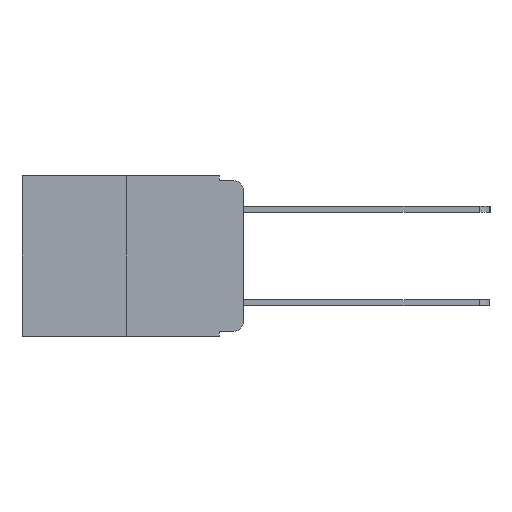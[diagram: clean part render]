
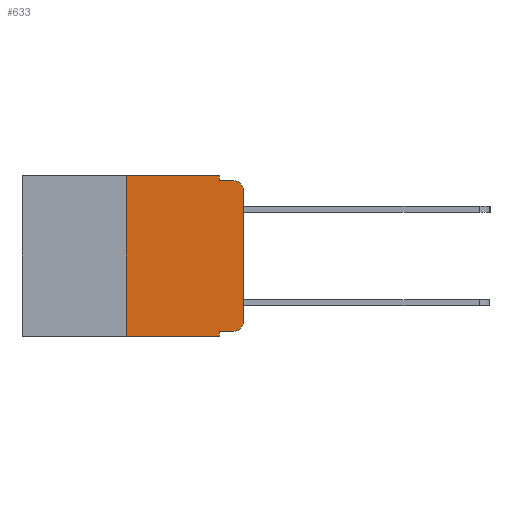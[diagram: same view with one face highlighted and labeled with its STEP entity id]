
A CAD part, left-side view. The second image highlights one B-rep face of the part: STEP entity #633.
In plain terms, the highlighted planar face has unit normal (-1, 0, 0).
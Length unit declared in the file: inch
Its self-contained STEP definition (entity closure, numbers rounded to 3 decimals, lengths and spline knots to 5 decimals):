
#31 = DIRECTION ( 'NONE',  ( 0., 0., -1. ) ) ;
#54 = DIRECTION ( 'NONE',  ( -1., 0., 0. ) ) ;
#389 = CARTESIAN_POINT ( 'NONE',  ( 0., 0.051, -0.333 ) ) ;
#633 = ADVANCED_FACE ( 'NONE', ( #2330 ), #4929, .F. ) ;
#895 = ORIENTED_EDGE ( 'NONE', *, *, #9284, .T. ) ;
#1005 = VERTEX_POINT ( 'NONE', #10512 ) ;
#1057 = ORIENTED_EDGE ( 'NONE', *, *, #10213, .T. ) ;
#1192 = CARTESIAN_POINT ( 'NONE',  ( 0., 0.051, 0. ) ) ;
#1267 = CARTESIAN_POINT ( 'NONE',  ( 0., 0.473, 0. ) ) ;
#1302 = VECTOR ( 'NONE', #1320, 39.37008 ) ;
#1320 = DIRECTION ( 'NONE',  ( 0., -1., 0. ) ) ;
#1490 = ORIENTED_EDGE ( 'NONE', *, *, #11199, .F. ) ;
#1569 = EDGE_CURVE ( 'NONE', #8359, #9452, #6798, .T. ) ;
#1632 = CARTESIAN_POINT ( 'NONE',  ( 0., 0.051, -0.343 ) ) ;
#1919 = ORIENTED_EDGE ( 'NONE', *, *, #7229, .T. ) ;
#2298 = VERTEX_POINT ( 'NONE', #8147 ) ;
#2330 = FACE_OUTER_BOUND ( 'NONE', #6310, .T. ) ;
#2711 = VERTEX_POINT ( 'NONE', #11053 ) ;
#2845 = CARTESIAN_POINT ( 'NONE',  ( 0., 0.02, -0.03 ) ) ;
#3116 = VECTOR ( 'NONE', #3587, 39.37008 ) ;
#3314 = DIRECTION ( 'NONE',  ( 0., 0., -1. ) ) ;
#3316 = DIRECTION ( 'NONE',  ( 1., 0., 0. ) ) ;
#3587 = DIRECTION ( 'NONE',  ( 0., -1., 0. ) ) ;
#3621 = LINE ( 'NONE', #7138, #10541 ) ;
#3807 = DIRECTION ( 'NONE',  ( 0., 0., -1. ) ) ;
#3878 = CIRCLE ( 'NONE', #7748, 0.02 ) ;
#3996 = LINE ( 'NONE', #1267, #10617 ) ;
#4294 = ORIENTED_EDGE ( 'NONE', *, *, #10607, .F. ) ;
#4360 = CARTESIAN_POINT ( 'NONE',  ( 0., 0., -0.313 ) ) ;
#4383 = ORIENTED_EDGE ( 'NONE', *, *, #5489, .T. ) ;
#4604 = EDGE_CURVE ( 'NONE', #1005, #2711, #3621, .T. ) ;
#4820 = DIRECTION ( 'NONE',  ( 0., 0., 1. ) ) ;
#4922 = VERTEX_POINT ( 'NONE', #10764 ) ;
#4929 = PLANE ( 'NONE',  #8745 ) ;
#5046 = VECTOR ( 'NONE', #6000, 39.37008 ) ;
#5053 = LINE ( 'NONE', #1192, #9042 ) ;
#5391 = LINE ( 'NONE', #9741, #10130 ) ;
#5489 = EDGE_CURVE ( 'NONE', #9452, #8325, #3878, .T. ) ;
#5541 = CARTESIAN_POINT ( 'NONE',  ( 0., 0.473, -0.343 ) ) ;
#5900 = EDGE_CURVE ( 'NONE', #8359, #11539, #7569, .T. ) ;
#6000 = DIRECTION ( 'NONE',  ( 0., 0., -1. ) ) ;
#6018 = CARTESIAN_POINT ( 'NONE',  ( 0., 0.051, 0. ) ) ;
#6022 = CARTESIAN_POINT ( 'NONE',  ( 0., 0.02, -0.333 ) ) ;
#6310 = EDGE_LOOP ( 'NONE', ( #895, #1057, #4294, #1490, #11759, #9511, #1919, #7731, #10321, #4383 ) ) ;
#6686 = LINE ( 'NONE', #10192, #9015 ) ;
#6798 = LINE ( 'NONE', #8460, #1302 ) ;
#7138 = CARTESIAN_POINT ( 'NONE',  ( 0., 0.25, 0. ) ) ;
#7229 = EDGE_CURVE ( 'NONE', #1005, #11539, #10396, .T. ) ;
#7234 = CARTESIAN_POINT ( 'NONE',  ( 0., 0., -0.03 ) ) ;
#7350 = DIRECTION ( 'NONE',  ( 0., 0., 1. ) ) ;
#7569 = LINE ( 'NONE', #6018, #5046 ) ;
#7731 = ORIENTED_EDGE ( 'NONE', *, *, #5900, .F. ) ;
#7748 = AXIS2_PLACEMENT_3D ( 'NONE', #10839, #54, #31 ) ;
#7845 = AXIS2_PLACEMENT_3D ( 'NONE', #2845, #9283, #3807 ) ;
#8147 = CARTESIAN_POINT ( 'NONE',  ( 0., 0.051, -0.01 ) ) ;
#8325 = VERTEX_POINT ( 'NONE', #4360 ) ;
#8359 = VERTEX_POINT ( 'NONE', #389 ) ;
#8460 = CARTESIAN_POINT ( 'NONE',  ( 0., 0.051, -0.333 ) ) ;
#8745 = AXIS2_PLACEMENT_3D ( 'NONE', #10022, #3316, #3314 ) ;
#8822 = DIRECTION ( 'NONE',  ( 0., -1., 0. ) ) ;
#8931 = VERTEX_POINT ( 'NONE', #7234 ) ;
#9015 = VECTOR ( 'NONE', #4820, 39.37008 ) ;
#9042 = VECTOR ( 'NONE', #10545, 39.37008 ) ;
#9283 = DIRECTION ( 'NONE',  ( -1., 0., 0. ) ) ;
#9284 = EDGE_CURVE ( 'NONE', #8325, #8931, #6686, .T. ) ;
#9452 = VERTEX_POINT ( 'NONE', #6022 ) ;
#9511 = ORIENTED_EDGE ( 'NONE', *, *, #4604, .F. ) ;
#9741 = CARTESIAN_POINT ( 'NONE',  ( 0., 0.051, -0.01 ) ) ;
#9833 = CARTESIAN_POINT ( 'NONE',  ( 0., 0.02, -0.01 ) ) ;
#10022 = CARTESIAN_POINT ( 'NONE',  ( 0., 0.473, 0. ) ) ;
#10130 = VECTOR ( 'NONE', #11449, 39.37008 ) ;
#10137 = CIRCLE ( 'NONE', #7845, 0.02 ) ;
#10192 = CARTESIAN_POINT ( 'NONE',  ( 0., 0., 0. ) ) ;
#10213 = EDGE_CURVE ( 'NONE', #8931, #11391, #10137, .T. ) ;
#10321 = ORIENTED_EDGE ( 'NONE', *, *, #1569, .T. ) ;
#10396 = LINE ( 'NONE', #5541, #3116 ) ;
#10512 = CARTESIAN_POINT ( 'NONE',  ( 0., 0.25, -0.343 ) ) ;
#10541 = VECTOR ( 'NONE', #7350, 39.37008 ) ;
#10545 = DIRECTION ( 'NONE',  ( 0., 0., -1. ) ) ;
#10607 = EDGE_CURVE ( 'NONE', #2298, #11391, #5391, .T. ) ;
#10617 = VECTOR ( 'NONE', #8822, 39.37008 ) ;
#10764 = CARTESIAN_POINT ( 'NONE',  ( 0., 0.051, 0. ) ) ;
#10839 = CARTESIAN_POINT ( 'NONE',  ( 0., 0.02, -0.313 ) ) ;
#11053 = CARTESIAN_POINT ( 'NONE',  ( 0., 0.25, 0. ) ) ;
#11199 = EDGE_CURVE ( 'NONE', #4922, #2298, #5053, .T. ) ;
#11391 = VERTEX_POINT ( 'NONE', #9833 ) ;
#11449 = DIRECTION ( 'NONE',  ( 0., -1., 0. ) ) ;
#11539 = VERTEX_POINT ( 'NONE', #1632 ) ;
#11759 = ORIENTED_EDGE ( 'NONE', *, *, #12066, .F. ) ;
#12066 = EDGE_CURVE ( 'NONE', #2711, #4922, #3996, .T. ) ;
